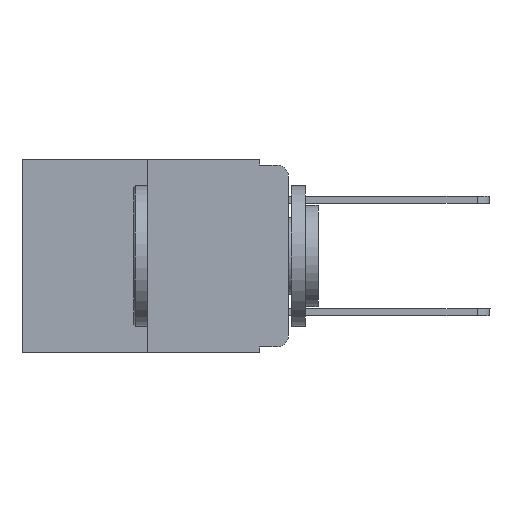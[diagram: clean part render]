
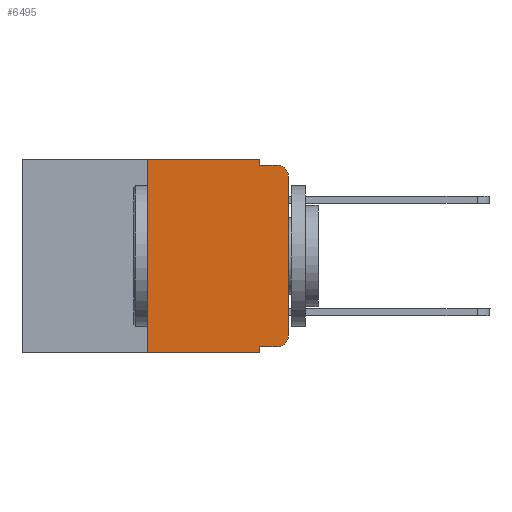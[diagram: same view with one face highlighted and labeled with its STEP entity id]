
A CAD part, left-side view. The second image highlights one B-rep face of the part: STEP entity #6495.
In plain terms, the highlighted planar face has unit normal (-1, 0, 0).
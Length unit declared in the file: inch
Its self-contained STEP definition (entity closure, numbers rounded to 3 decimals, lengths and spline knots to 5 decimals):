
#249 = DIRECTION ( 'NONE',  ( 0., 0., -1. ) ) ;
#270 = LINE ( 'NONE', #5922, #12087 ) ;
#361 = CARTESIAN_POINT ( 'NONE',  ( 0., 0.051, 0. ) ) ;
#496 = VERTEX_POINT ( 'NONE', #2957 ) ;
#497 = CARTESIAN_POINT ( 'NONE',  ( 0., 0.051, -0.333 ) ) ;
#540 = CARTESIAN_POINT ( 'NONE',  ( 0., 0.02, -0.333 ) ) ;
#728 = VERTEX_POINT ( 'NONE', #6363 ) ;
#1079 = ORIENTED_EDGE ( 'NONE', *, *, #2276, .T. ) ;
#1253 = EDGE_CURVE ( 'NONE', #496, #3453, #5908, .T. ) ;
#1313 = LINE ( 'NONE', #9712, #3099 ) ;
#1481 = ORIENTED_EDGE ( 'NONE', *, *, #4698, .F. ) ;
#1777 = CARTESIAN_POINT ( 'NONE',  ( 0., 0.051, -0.01 ) ) ;
#2276 = EDGE_CURVE ( 'NONE', #6263, #728, #5875, .T. ) ;
#2384 = AXIS2_PLACEMENT_3D ( 'NONE', #2452, #8186, #6891 ) ;
#2418 = ORIENTED_EDGE ( 'NONE', *, *, #11795, .F. ) ;
#2442 = EDGE_CURVE ( 'NONE', #496, #8923, #7199, .T. ) ;
#2452 = CARTESIAN_POINT ( 'NONE',  ( 0., 0.02, -0.313 ) ) ;
#2517 = EDGE_LOOP ( 'NONE', ( #7731, #1079, #1481, #17959, #7922, #4414, #12157, #2418, #3554, #13115 ) ) ;
#2525 = EDGE_CURVE ( 'NONE', #10134, #10597, #270, .T. ) ;
#2550 = EDGE_CURVE ( 'NONE', #11747, #4362, #10283, .T. ) ;
#2633 = CARTESIAN_POINT ( 'NONE',  ( 0., 0.473, 0. ) ) ;
#2720 = VECTOR ( 'NONE', #8642, 39.37008 ) ;
#2875 = DIRECTION ( 'NONE',  ( 0., 0., -1. ) ) ;
#2957 = CARTESIAN_POINT ( 'NONE',  ( 0., 0.25, -0.343 ) ) ;
#3012 = LINE ( 'NONE', #12903, #13948 ) ;
#3099 = VECTOR ( 'NONE', #4071, 39.37008 ) ;
#3453 = VERTEX_POINT ( 'NONE', #8854 ) ;
#3554 = ORIENTED_EDGE ( 'NONE', *, *, #2525, .T. ) ;
#3615 = VECTOR ( 'NONE', #249, 39.37008 ) ;
#3883 = CIRCLE ( 'NONE', #2384, 0.02 ) ;
#3893 = CARTESIAN_POINT ( 'NONE',  ( 0., 0., -0.03 ) ) ;
#4071 = DIRECTION ( 'NONE',  ( 0., -1., 0. ) ) ;
#4290 = VERTEX_POINT ( 'NONE', #13256 ) ;
#4293 = AXIS2_PLACEMENT_3D ( 'NONE', #17897, #13764, #9336 ) ;
#4362 = VERTEX_POINT ( 'NONE', #1777 ) ;
#4414 = ORIENTED_EDGE ( 'NONE', *, *, #2442, .F. ) ;
#4698 = EDGE_CURVE ( 'NONE', #4362, #728, #1313, .T. ) ;
#5757 = DIRECTION ( 'NONE',  ( 0., -1., 0. ) ) ;
#5875 = CIRCLE ( 'NONE', #4293, 0.02 ) ;
#5908 = LINE ( 'NONE', #17891, #7255 ) ;
#5922 = CARTESIAN_POINT ( 'NONE',  ( 0., 0.051, -0.333 ) ) ;
#6263 = VERTEX_POINT ( 'NONE', #3893 ) ;
#6363 = CARTESIAN_POINT ( 'NONE',  ( 0., 0.02, -0.01 ) ) ;
#6495 = ADVANCED_FACE ( 'NONE', ( #16426 ), #6892, .F. ) ;
#6670 = EDGE_CURVE ( 'NONE', #8923, #11747, #3012, .T. ) ;
#6891 = DIRECTION ( 'NONE',  ( 0., 0., -1. ) ) ;
#6892 = PLANE ( 'NONE',  #11628 ) ;
#7013 = DIRECTION ( 'NONE',  ( 1., 0., 0. ) ) ;
#7199 = LINE ( 'NONE', #14201, #2720 ) ;
#7255 = VECTOR ( 'NONE', #13627, 39.37008 ) ;
#7422 = DIRECTION ( 'NONE',  ( 0., 0., 1. ) ) ;
#7731 = ORIENTED_EDGE ( 'NONE', *, *, #8515, .T. ) ;
#7922 = ORIENTED_EDGE ( 'NONE', *, *, #6670, .F. ) ;
#8044 = LINE ( 'NONE', #15997, #14948 ) ;
#8186 = DIRECTION ( 'NONE',  ( -1., 0., 0. ) ) ;
#8362 = DIRECTION ( 'NONE',  ( 0., 0., -1. ) ) ;
#8515 = EDGE_CURVE ( 'NONE', #4290, #6263, #8044, .T. ) ;
#8642 = DIRECTION ( 'NONE',  ( 0., 0., 1. ) ) ;
#8764 = DIRECTION ( 'NONE',  ( 0., -1., 0. ) ) ;
#8854 = CARTESIAN_POINT ( 'NONE',  ( 0., 0.051, -0.343 ) ) ;
#8923 = VERTEX_POINT ( 'NONE', #10640 ) ;
#9336 = DIRECTION ( 'NONE',  ( 0., 0., -1. ) ) ;
#9712 = CARTESIAN_POINT ( 'NONE',  ( 0., 0.051, -0.01 ) ) ;
#10134 = VERTEX_POINT ( 'NONE', #497 ) ;
#10283 = LINE ( 'NONE', #361, #3615 ) ;
#10597 = VERTEX_POINT ( 'NONE', #540 ) ;
#10640 = CARTESIAN_POINT ( 'NONE',  ( 0., 0.25, 0. ) ) ;
#11628 = AXIS2_PLACEMENT_3D ( 'NONE', #2633, #7013, #8362 ) ;
#11747 = VERTEX_POINT ( 'NONE', #16191 ) ;
#11795 = EDGE_CURVE ( 'NONE', #10134, #3453, #14379, .T. ) ;
#11939 = VECTOR ( 'NONE', #2875, 39.37008 ) ;
#12087 = VECTOR ( 'NONE', #8764, 39.37008 ) ;
#12157 = ORIENTED_EDGE ( 'NONE', *, *, #1253, .T. ) ;
#12753 = EDGE_CURVE ( 'NONE', #10597, #4290, #3883, .T. ) ;
#12903 = CARTESIAN_POINT ( 'NONE',  ( 0., 0.473, 0. ) ) ;
#13115 = ORIENTED_EDGE ( 'NONE', *, *, #12753, .T. ) ;
#13256 = CARTESIAN_POINT ( 'NONE',  ( 0., 0., -0.313 ) ) ;
#13627 = DIRECTION ( 'NONE',  ( 0., -1., 0. ) ) ;
#13764 = DIRECTION ( 'NONE',  ( -1., 0., 0. ) ) ;
#13948 = VECTOR ( 'NONE', #5757, 39.37008 ) ;
#14154 = CARTESIAN_POINT ( 'NONE',  ( 0., 0.051, 0. ) ) ;
#14201 = CARTESIAN_POINT ( 'NONE',  ( 0., 0.25, 0. ) ) ;
#14379 = LINE ( 'NONE', #14154, #11939 ) ;
#14948 = VECTOR ( 'NONE', #7422, 39.37008 ) ;
#15997 = CARTESIAN_POINT ( 'NONE',  ( 0., 0., 0. ) ) ;
#16191 = CARTESIAN_POINT ( 'NONE',  ( 0., 0.051, 0. ) ) ;
#16426 = FACE_OUTER_BOUND ( 'NONE', #2517, .T. ) ;
#17891 = CARTESIAN_POINT ( 'NONE',  ( 0., 0.473, -0.343 ) ) ;
#17897 = CARTESIAN_POINT ( 'NONE',  ( 0., 0.02, -0.03 ) ) ;
#17959 = ORIENTED_EDGE ( 'NONE', *, *, #2550, .F. ) ;
